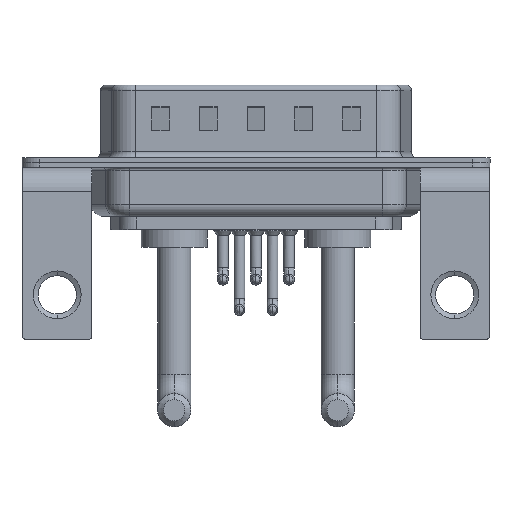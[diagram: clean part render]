
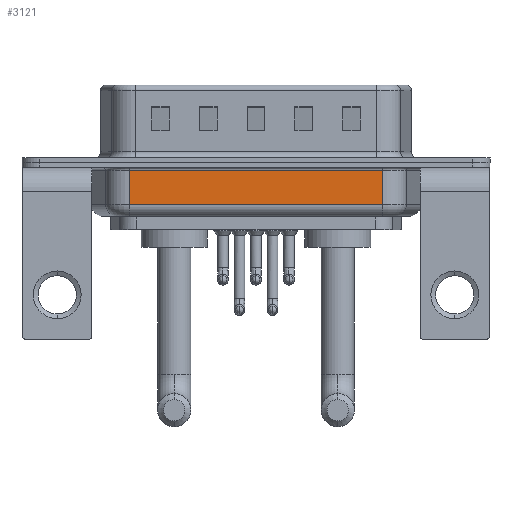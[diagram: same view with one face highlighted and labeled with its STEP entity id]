
A CAD part, front view. The second image highlights one B-rep face of the part: STEP entity #3121.
In plain terms, the highlighted planar face has unit normal (0, -1, 0).
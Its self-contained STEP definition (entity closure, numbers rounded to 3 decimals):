
#902 = EDGE_LOOP ( 'NONE', ( #5363, #3748, #4142, #17415 ) ) ;
#2558 = PLANE ( 'NONE',  #8326 ) ;
#3121 = ADVANCED_FACE ( 'NONE', ( #21060 ), #2558, .F. ) ;
#3748 = ORIENTED_EDGE ( 'NONE', *, *, #20111, .T. ) ;
#4142 = ORIENTED_EDGE ( 'NONE', *, *, #15583, .T. ) ;
#4154 = CARTESIAN_POINT ( 'NONE',  ( 27.269, -5.35, -4.5 ) ) ;
#4518 = VERTEX_POINT ( 'NONE', #19742 ) ;
#4991 = VERTEX_POINT ( 'NONE', #13179 ) ;
#5363 = ORIENTED_EDGE ( 'NONE', *, *, #5698, .F. ) ;
#5570 = DIRECTION ( 'NONE',  ( 0., 0., 1. ) ) ;
#5698 = EDGE_CURVE ( 'NONE', #4518, #7508, #14103, .T. ) ;
#6193 = LINE ( 'NONE', #12965, #13600 ) ;
#7508 = VERTEX_POINT ( 'NONE', #16486 ) ;
#8326 = AXIS2_PLACEMENT_3D ( 'NONE', #9327, #20736, #5570 ) ;
#9327 = CARTESIAN_POINT ( 'NONE',  ( 6.031, -5.35, -4.5 ) ) ;
#9688 = DIRECTION ( 'NONE',  ( 1., 0., 0. ) ) ;
#9723 = VERTEX_POINT ( 'NONE', #10250 ) ;
#10250 = CARTESIAN_POINT ( 'NONE',  ( 27.269, -5.35, -3.5 ) ) ;
#11439 = VECTOR ( 'NONE', #17426, 1000. ) ;
#12481 = DIRECTION ( 'NONE',  ( 0., 0., 1. ) ) ;
#12965 = CARTESIAN_POINT ( 'NONE',  ( 6.031, -5.35, -0.65 ) ) ;
#13179 = CARTESIAN_POINT ( 'NONE',  ( 27.269, -5.35, -0.65 ) ) ;
#13600 = VECTOR ( 'NONE', #19695, 1000. ) ;
#14103 = LINE ( 'NONE', #15870, #11439 ) ;
#14910 = EDGE_CURVE ( 'NONE', #4991, #7508, #6193, .T. ) ;
#15583 = EDGE_CURVE ( 'NONE', #9723, #4991, #20986, .T. ) ;
#15870 = CARTESIAN_POINT ( 'NONE',  ( 6.031, -5.35, -4.5 ) ) ;
#16486 = CARTESIAN_POINT ( 'NONE',  ( 6.031, -5.35, -0.65 ) ) ;
#16786 = VECTOR ( 'NONE', #12481, 1000. ) ;
#17415 = ORIENTED_EDGE ( 'NONE', *, *, #14910, .T. ) ;
#17426 = DIRECTION ( 'NONE',  ( 0., 0., 1. ) ) ;
#17774 = VECTOR ( 'NONE', #9688, 1000. ) ;
#18230 = CARTESIAN_POINT ( 'NONE',  ( 6.031, -5.35, -3.5 ) ) ;
#19695 = DIRECTION ( 'NONE',  ( -1., 0., 0. ) ) ;
#19742 = CARTESIAN_POINT ( 'NONE',  ( 6.031, -5.35, -3.5 ) ) ;
#20111 = EDGE_CURVE ( 'NONE', #4518, #9723, #21502, .T. ) ;
#20736 = DIRECTION ( 'NONE',  ( 0., 1., 0. ) ) ;
#20986 = LINE ( 'NONE', #4154, #16786 ) ;
#21060 = FACE_OUTER_BOUND ( 'NONE', #902, .T. ) ;
#21502 = LINE ( 'NONE', #18230, #17774 ) ;
